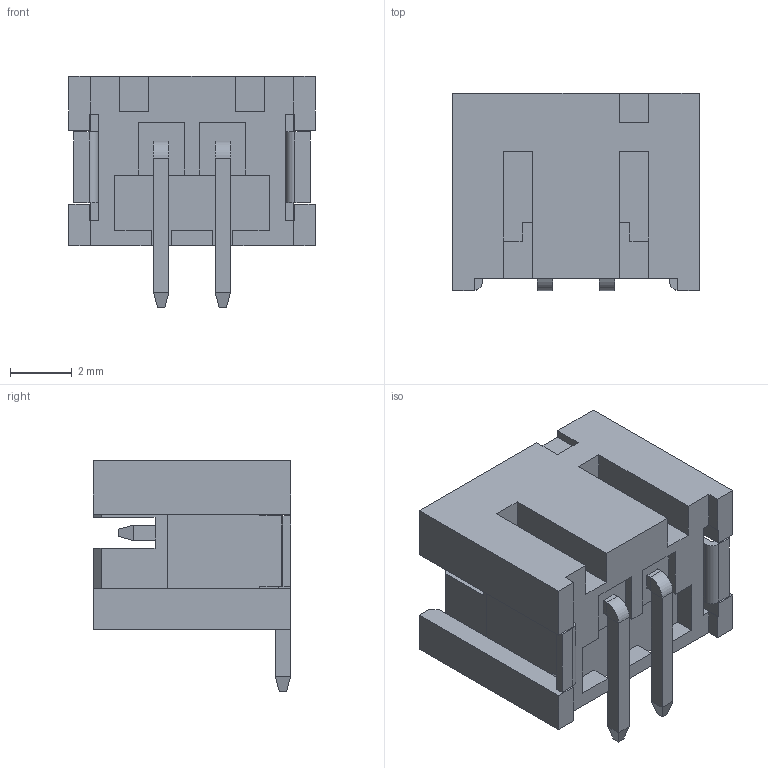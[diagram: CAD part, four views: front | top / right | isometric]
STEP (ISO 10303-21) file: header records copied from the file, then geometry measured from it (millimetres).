
FILE_DESCRIPTION (( 'STEP AP203' ), '1' );
FILE_NAME ('140-502-417-011.STEP', '2020-03-31T20:00:50', ( '' ), ( '' ), 'SwSTEP 2.0', 'SolidWorks 2016', '' );
FILE_SCHEMA (( 'CONFIG_CONTROL_DESIGN' ));
Length unit declared in the file: millimetre
Products named in the file (4): 140-502-417-011; V SMT Contact; V SMT Housing_502; V SMT Pad
Assembly tree (5 placements, depth 2):
  140-502-417-011
    V SMT Housing_502
    V SMT Contact  x2
    V SMT Pad  x2
Bounding box: 8 x 6.4 x 7.5 mm (x, y, z)
Volume: 145.2 mm3; surface area: 511 mm2
Topology: 5 solids, 5 shells, 176 faces, 468 edges, 298 vertices
Faces by surface type: plane 168, cylinder 8
Entity records: 4846 total; most frequent: CARTESIAN_POINT 786, ORIENTED_EDGE 776, DIRECTION 692, EDGE_CURVE 388, LINE 380, VECTOR 380, VERTEX_POINT 250, AXIS2_PLACEMENT_3D 156
